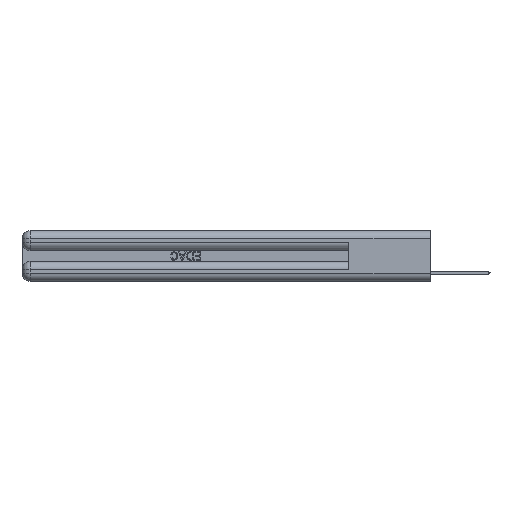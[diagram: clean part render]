
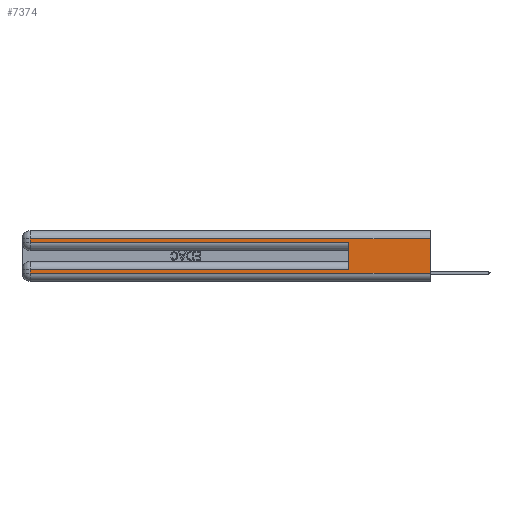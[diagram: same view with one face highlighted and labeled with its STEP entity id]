
A CAD part, left-side view. The second image highlights one B-rep face of the part: STEP entity #7374.
In plain terms, the highlighted planar face has unit normal (-1, 0, 0).
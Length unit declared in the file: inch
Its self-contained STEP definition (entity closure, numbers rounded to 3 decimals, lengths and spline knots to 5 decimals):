
#587 = LINE ( 'NONE', #24420, #905 ) ;
#662 = VECTOR ( 'NONE', #19742, 39.37008 ) ;
#905 = VECTOR ( 'NONE', #1407, 39.37008 ) ;
#1256 = LINE ( 'NONE', #11297, #17776 ) ;
#1407 = DIRECTION ( 'NONE',  ( 0., 1., 0. ) ) ;
#1588 = VERTEX_POINT ( 'NONE', #2337 ) ;
#2337 = CARTESIAN_POINT ( 'NONE',  ( 0., 2.94, 0.085 ) ) ;
#2677 = EDGE_CURVE ( 'NONE', #14228, #17269, #11753, .T. ) ;
#4421 = ORIENTED_EDGE ( 'NONE', *, *, #23937, .F. ) ;
#4553 = VERTEX_POINT ( 'NONE', #10182 ) ;
#5253 = CARTESIAN_POINT ( 'NONE',  ( 0., 0., 0.285 ) ) ;
#5307 = VECTOR ( 'NONE', #26124, 39.37008 ) ;
#5532 = ORIENTED_EDGE ( 'NONE', *, *, #22631, .T. ) ;
#5970 = LINE ( 'NONE', #5253, #5307 ) ;
#6318 = CARTESIAN_POINT ( 'NONE',  ( 0., 0.6, 0.145 ) ) ;
#7041 = EDGE_CURVE ( 'NONE', #10826, #1588, #25228, .T. ) ;
#7165 = VERTEX_POINT ( 'NONE', #13860 ) ;
#7249 = DIRECTION ( 'NONE',  ( 1., 0., 0. ) ) ;
#7315 = CARTESIAN_POINT ( 'NONE',  ( 0., 2.94, 0.37 ) ) ;
#7374 = ADVANCED_FACE ( 'NONE', ( #15941 ), #15552, .F. ) ;
#8287 = CARTESIAN_POINT ( 'NONE',  ( 0., 0.6, 0.285 ) ) ;
#8475 = DIRECTION ( 'NONE',  ( 0., -1., 0. ) ) ;
#8711 = EDGE_CURVE ( 'NONE', #17269, #20609, #5970, .T. ) ;
#8813 = CARTESIAN_POINT ( 'NONE',  ( 0., 2.94, 0.37 ) ) ;
#10182 = CARTESIAN_POINT ( 'NONE',  ( 0., 2.94, 0.06 ) ) ;
#10404 = EDGE_CURVE ( 'NONE', #13864, #14228, #587, .T. ) ;
#10826 = VERTEX_POINT ( 'NONE', #13435 ) ;
#11297 = CARTESIAN_POINT ( 'NONE',  ( 0., 0., 0.37 ) ) ;
#11753 = LINE ( 'NONE', #7315, #21669 ) ;
#11859 = EDGE_CURVE ( 'NONE', #10826, #20609, #22309, .T. ) ;
#12187 = DIRECTION ( 'NONE',  ( 0., 1., 0. ) ) ;
#13322 = EDGE_CURVE ( 'NONE', #4553, #7165, #17357, .T. ) ;
#13435 = CARTESIAN_POINT ( 'NONE',  ( 0., 0.6, 0.085 ) ) ;
#13622 = DIRECTION ( 'NONE',  ( 0., 0., -1. ) ) ;
#13723 = ORIENTED_EDGE ( 'NONE', *, *, #10404, .T. ) ;
#13776 = DIRECTION ( 'NONE',  ( 0., 0., -1. ) ) ;
#13812 = CARTESIAN_POINT ( 'NONE',  ( 0., 2.94, 0.285 ) ) ;
#13860 = CARTESIAN_POINT ( 'NONE',  ( 0., 0., 0.06 ) ) ;
#13864 = VERTEX_POINT ( 'NONE', #19259 ) ;
#14228 = VERTEX_POINT ( 'NONE', #23475 ) ;
#14319 = ORIENTED_EDGE ( 'NONE', *, *, #11859, .F. ) ;
#14431 = VECTOR ( 'NONE', #8475, 39.37008 ) ;
#14725 = VECTOR ( 'NONE', #23244, 39.37008 ) ;
#15552 = PLANE ( 'NONE',  #18935 ) ;
#15861 = LINE ( 'NONE', #8813, #662 ) ;
#15941 = FACE_OUTER_BOUND ( 'NONE', #21418, .T. ) ;
#17269 = VERTEX_POINT ( 'NONE', #13812 ) ;
#17357 = LINE ( 'NONE', #21102, #14431 ) ;
#17776 = VECTOR ( 'NONE', #26050, 39.37008 ) ;
#18443 = ORIENTED_EDGE ( 'NONE', *, *, #2677, .T. ) ;
#18935 = AXIS2_PLACEMENT_3D ( 'NONE', #21578, #7249, #13622 ) ;
#19259 = CARTESIAN_POINT ( 'NONE',  ( 0., 0., 0.31 ) ) ;
#19742 = DIRECTION ( 'NONE',  ( 0., 0., -1. ) ) ;
#20124 = ORIENTED_EDGE ( 'NONE', *, *, #7041, .T. ) ;
#20308 = ORIENTED_EDGE ( 'NONE', *, *, #8711, .T. ) ;
#20609 = VERTEX_POINT ( 'NONE', #8287 ) ;
#21102 = CARTESIAN_POINT ( 'NONE',  ( 0., 0., 0.06 ) ) ;
#21418 = EDGE_LOOP ( 'NONE', ( #4421, #13723, #18443, #20308, #14319, #20124, #5532, #25491 ) ) ;
#21578 = CARTESIAN_POINT ( 'NONE',  ( 0., 0., 0.37 ) ) ;
#21669 = VECTOR ( 'NONE', #13776, 39.37008 ) ;
#22309 = LINE ( 'NONE', #6318, #14725 ) ;
#22631 = EDGE_CURVE ( 'NONE', #1588, #4553, #15861, .T. ) ;
#23244 = DIRECTION ( 'NONE',  ( 0., 0., 1. ) ) ;
#23475 = CARTESIAN_POINT ( 'NONE',  ( 0., 2.94, 0.31 ) ) ;
#23937 = EDGE_CURVE ( 'NONE', #13864, #7165, #1256, .T. ) ;
#24420 = CARTESIAN_POINT ( 'NONE',  ( 0., 0., 0.31 ) ) ;
#24747 = CARTESIAN_POINT ( 'NONE',  ( 0., 0., 0.085 ) ) ;
#25228 = LINE ( 'NONE', #24747, #26843 ) ;
#25491 = ORIENTED_EDGE ( 'NONE', *, *, #13322, .T. ) ;
#26050 = DIRECTION ( 'NONE',  ( 0., 0., -1. ) ) ;
#26124 = DIRECTION ( 'NONE',  ( 0., -1., 0. ) ) ;
#26843 = VECTOR ( 'NONE', #12187, 39.37008 ) ;
